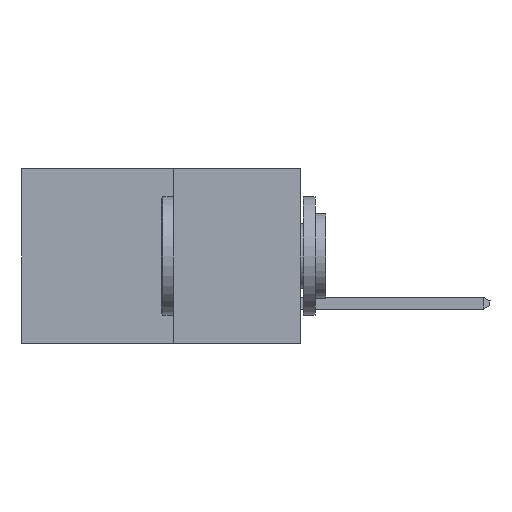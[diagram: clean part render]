
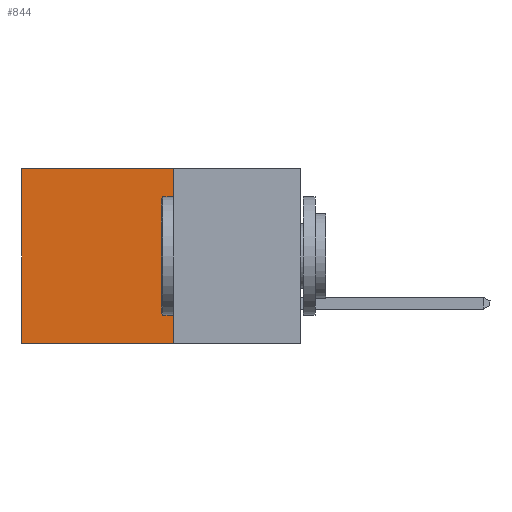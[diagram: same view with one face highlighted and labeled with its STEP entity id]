
A CAD part, left-side view. The second image highlights one B-rep face of the part: STEP entity #844.
In plain terms, the highlighted planar face has unit normal (-1, 0, 0).
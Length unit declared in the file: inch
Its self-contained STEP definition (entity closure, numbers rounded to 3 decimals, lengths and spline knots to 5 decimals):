
#208 = DIRECTION ( 'NONE',  ( 0., 0., -1. ) ) ;
#587 = DIRECTION ( 'NONE',  ( 0., 1., 0. ) ) ;
#681 = CARTESIAN_POINT ( 'NONE',  ( 0.277, 0.27, -0.37 ) ) ;
#844 = ADVANCED_FACE ( 'NONE', ( #8517 ), #4245, .F. ) ;
#1006 = EDGE_CURVE ( 'NONE', #12936, #1148, #7620, .T. ) ;
#1148 = VERTEX_POINT ( 'NONE', #10690 ) ;
#1153 = ORIENTED_EDGE ( 'NONE', *, *, #8454, .F. ) ;
#1843 = EDGE_CURVE ( 'NONE', #9404, #12727, #14247, .T. ) ;
#2895 = ORIENTED_EDGE ( 'NONE', *, *, #1006, .F. ) ;
#4226 = DIRECTION ( 'NONE',  ( 1., 0., 0. ) ) ;
#4245 = PLANE ( 'NONE',  #9934 ) ;
#4441 = VECTOR ( 'NONE', #587, 39.37008 ) ;
#4463 = CARTESIAN_POINT ( 'NONE',  ( 0.277, 0.27, -0.37 ) ) ;
#6218 = DIRECTION ( 'NONE',  ( 0., 0., -1. ) ) ;
#6741 = CARTESIAN_POINT ( 'NONE',  ( 0.277, 0.27, -0.37 ) ) ;
#7620 = LINE ( 'NONE', #6741, #4441 ) ;
#8116 = LINE ( 'NONE', #681, #13704 ) ;
#8127 = LINE ( 'NONE', #9619, #14067 ) ;
#8454 = EDGE_CURVE ( 'NONE', #9404, #12936, #8116, .T. ) ;
#8517 = FACE_OUTER_BOUND ( 'NONE', #14482, .T. ) ;
#8775 = CARTESIAN_POINT ( 'NONE',  ( 0.277, 0.27, -0.37 ) ) ;
#9404 = VERTEX_POINT ( 'NONE', #14354 ) ;
#9619 = CARTESIAN_POINT ( 'NONE',  ( 0.277, 0.59, -0.37 ) ) ;
#9934 = AXIS2_PLACEMENT_3D ( 'NONE', #4463, #4226, #13758 ) ;
#10553 = EDGE_CURVE ( 'NONE', #12727, #1148, #8127, .T. ) ;
#10690 = CARTESIAN_POINT ( 'NONE',  ( 0.277, 0.59, -0.37 ) ) ;
#11182 = ORIENTED_EDGE ( 'NONE', *, *, #1843, .T. ) ;
#11274 = VECTOR ( 'NONE', #11519, 39.37008 ) ;
#11519 = DIRECTION ( 'NONE',  ( 0., 1., 0. ) ) ;
#12067 = CARTESIAN_POINT ( 'NONE',  ( 0.277, 0.59, 0. ) ) ;
#12579 = CARTESIAN_POINT ( 'NONE',  ( 0.277, 0.27, 0. ) ) ;
#12727 = VERTEX_POINT ( 'NONE', #12067 ) ;
#12936 = VERTEX_POINT ( 'NONE', #8775 ) ;
#13191 = ORIENTED_EDGE ( 'NONE', *, *, #10553, .T. ) ;
#13704 = VECTOR ( 'NONE', #208, 39.37008 ) ;
#13758 = DIRECTION ( 'NONE',  ( 0., 0., -1. ) ) ;
#14067 = VECTOR ( 'NONE', #6218, 39.37008 ) ;
#14247 = LINE ( 'NONE', #12579, #11274 ) ;
#14354 = CARTESIAN_POINT ( 'NONE',  ( 0.277, 0.27, 0. ) ) ;
#14482 = EDGE_LOOP ( 'NONE', ( #13191, #2895, #1153, #11182 ) ) ;
